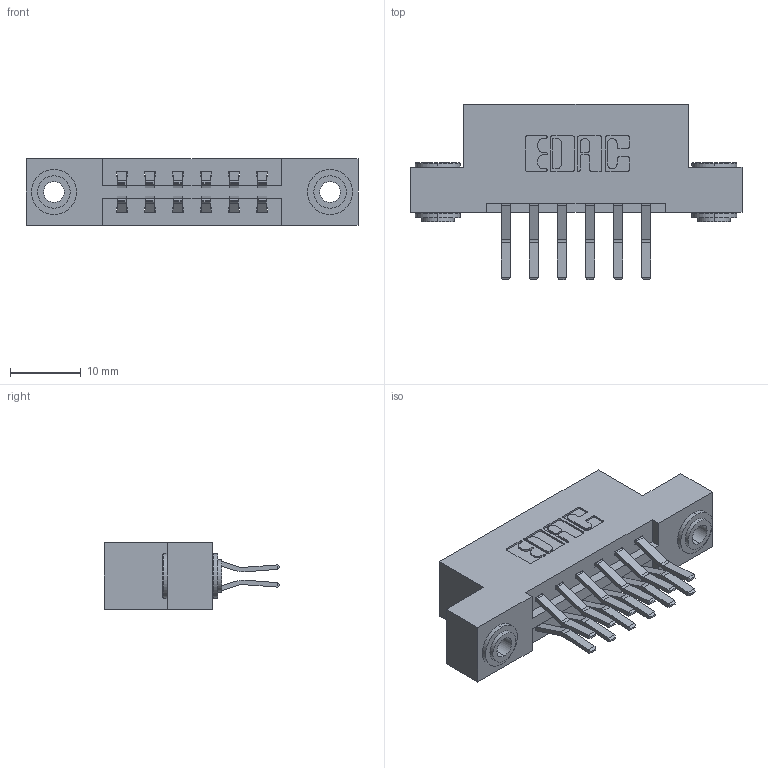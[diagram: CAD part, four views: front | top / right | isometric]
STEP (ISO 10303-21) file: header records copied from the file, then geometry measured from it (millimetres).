
FILE_DESCRIPTION (( 'STEP AP203' ), '1' );
FILE_NAME ('337-012-560-203.STEP', '2019-10-08T11:26:31', ( '' ), ( '' ), 'SwSTEP 2.0', 'SolidWorks 2016', '' );
FILE_SCHEMA (( 'CONFIG_CONTROL_DESIGN' ));
Length unit declared in the file: inch
Products named in the file (4): 337 Part_Flush Mounting Lugs - 0.156 Dia-TH; 345-292-001_560 Tail; 337-012-560-203; 345-250-002_345-250-002-102
Assembly tree (15 placements, depth 2):
  337-012-560-203
    337 Part_Flush Mounting Lugs - 0.156 Dia-TH
    345-292-001_560 Tail  x12
    345-250-002_345-250-002-102  x2
Bounding box: 46.79 x 24.78 x 9.4 mm (x, y, z)
Volume: 4549.6 mm3; surface area: 5245.7 mm2
Topology: 15 solids, 15 shells, 824 faces, 2391 edges, 1574 vertices
Faces by surface type: plane 536, cylinder 280, cone 8
Entity records: 10046 total; most frequent: CARTESIAN_POINT 1697, ORIENTED_EDGE 1626, DIRECTION 1547, EDGE_CURVE 813, LINE 657, VECTOR 657, VERTEX_POINT 538, AXIS2_PLACEMENT_3D 445
